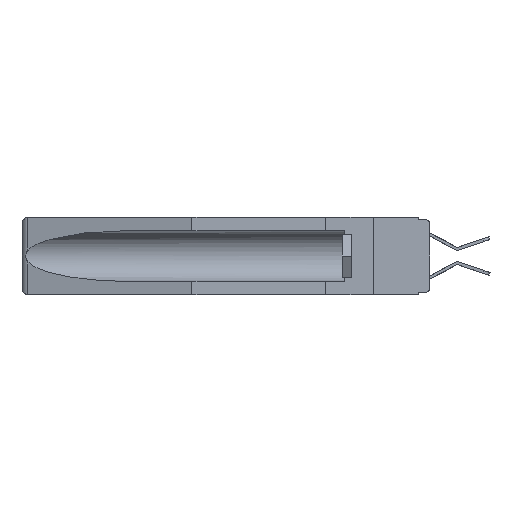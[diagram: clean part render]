
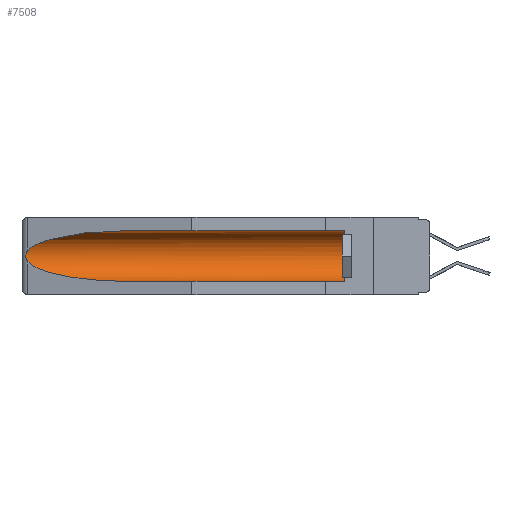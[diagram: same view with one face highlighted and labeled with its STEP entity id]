
A CAD part, left-side view. The second image highlights one B-rep face of the part: STEP entity #7508.
In plain terms, the highlighted cylindrical face has radius 2.857 mm (diameter 5.715 mm), a partial arc.
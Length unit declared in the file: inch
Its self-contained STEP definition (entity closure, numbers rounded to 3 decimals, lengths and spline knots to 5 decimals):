
#489 = CARTESIAN_POINT ( 'NONE',  ( 0.26655, 1.53094, -0.18657 ) ) ;
#800 = VERTEX_POINT ( 'NONE', #11729 ) ;
#881 = CARTESIAN_POINT ( 'NONE',  ( 0.26537, 1.52718, -0.14972 ) ) ;
#1043 = ORIENTED_EDGE ( 'NONE', *, *, #3522, .T. ) ;
#1989 = DIRECTION ( 'NONE',  ( 0., -1., 0. ) ) ;
#3190 = LINE ( 'NONE', #11113, #18363 ) ;
#3226 = CARTESIAN_POINT ( 'NONE',  ( 0.21114, 1.30732, -0.059 ) ) ;
#3404 = CARTESIAN_POINT ( 'NONE',  ( 0.155, 1.07973, -0.284 ) ) ;
#3522 = EDGE_CURVE ( 'NONE', #16618, #800, #25748, .T. ) ;
#3600 = CARTESIAN_POINT ( 'NONE',  ( 0.155, -0.30754, -0.1715 ) ) ;
#3727 = DIRECTION ( 'NONE',  ( 0., 0., 1. ) ) ;
#4139 = CARTESIAN_POINT ( 'NONE',  ( 0.155, 0.126, -0.284 ) ) ;
#4803 = EDGE_CURVE ( 'NONE', #12986, #12432, #3190, .T. ) ;
#4884 = CARTESIAN_POINT ( 'NONE',  ( 0.25451, 1.48313, -0.24835 ) ) ;
#6074 = AXIS2_PLACEMENT_3D ( 'NONE', #23642, #1989, #25483 ) ;
#6491 = CARTESIAN_POINT ( 'NONE',  ( 0.26654, 1.53092, -0.15636 ) ) ;
#6821 = EDGE_LOOP ( 'NONE', ( #10138, #25064, #18909, #18892, #12459, #1043 ) ) ;
#7356 = CARTESIAN_POINT ( 'NONE',  ( 0.155, -0.30754, -0.059 ) ) ;
#7508 = ADVANCED_FACE ( 'NONE', ( #21339 ), #17936, .F. ) ;
#8576 = CARTESIAN_POINT ( 'NONE',  ( 0.26597, 1.5296, -0.19026 ) ) ;
#9327 = CARTESIAN_POINT ( 'NONE',  ( 0.155, 1.07973, -0.059 ) ) ;
#10138 = ORIENTED_EDGE ( 'NONE', *, *, #19722, .T. ) ;
#10212 = CARTESIAN_POINT ( 'NONE',  ( 0.26537, 1.52718, -0.19328 ) ) ;
#11113 = CARTESIAN_POINT ( 'NONE',  ( 0.155, -0.30754, -0.284 ) ) ;
#11729 = CARTESIAN_POINT ( 'NONE',  ( 0.155, 1.07973, -0.059 ) ) ;
#12090 = VECTOR ( 'NONE', #21546, 39.37008 ) ;
#12373 = EDGE_CURVE ( 'NONE', #23852, #12432, #17902, .T. ) ;
#12432 = VERTEX_POINT ( 'NONE', #3404 ) ;
#12459 = ORIENTED_EDGE ( 'NONE', *, *, #13884, .T. ) ;
#12473 = CARTESIAN_POINT ( 'NONE',  ( 0.2675, 1.53308, -0.17534 ) ) ;
#12733 = CARTESIAN_POINT ( 'NONE',  ( 0.2673, 1.5327, -0.16383 ) ) ;
#12986 = VERTEX_POINT ( 'NONE', #4139 ) ;
#13369 = CARTESIAN_POINT ( 'NONE',  ( 0.26537, 1.52718, -0.14972 ) ) ;
#13410 =( BOUNDED_CURVE ( )  B_SPLINE_CURVE ( 3, ( #9327, #3226, #23426, #13369 ),
 .UNSPECIFIED., .F., .F. ) 
 B_SPLINE_CURVE_WITH_KNOTS ( ( 4, 4 ),
 ( 4.71239, 6.08839 ),
 .UNSPECIFIED. ) 
 CURVE ( )  GEOMETRIC_REPRESENTATION_ITEM ( )  RATIONAL_B_SPLINE_CURVE ( ( 1., 0.848, 0.848, 1. ) ) 
 REPRESENTATION_ITEM ( '' )  );
#13884 = EDGE_CURVE ( 'NONE', #12986, #16618, #17296, .T. ) ;
#15513 = AXIS2_PLACEMENT_3D ( 'NONE', #3600, #21589, #3727 ) ;
#15522 = VERTEX_POINT ( 'NONE', #24870 ) ;
#16386 = CARTESIAN_POINT ( 'NONE',  ( 0.2673, 1.53269, -0.17917 ) ) ;
#16521 = CARTESIAN_POINT ( 'NONE',  ( 0.26537, 1.52718, -0.19328 ) ) ;
#16618 = VERTEX_POINT ( 'NONE', #18069 ) ;
#17296 = CIRCLE ( 'NONE', #6074, 0.1125 ) ;
#17902 =( BOUNDED_CURVE ( )  B_SPLINE_CURVE ( 3, ( #23478, #4884, #19177, #23355 ),
 .UNSPECIFIED., .F., .F. ) 
 B_SPLINE_CURVE_WITH_KNOTS ( ( 4, 4 ),
 ( 0.1948, 1.5708 ),
 .UNSPECIFIED. ) 
 CURVE ( )  GEOMETRIC_REPRESENTATION_ITEM ( )  RATIONAL_B_SPLINE_CURVE ( ( 1., 0.848, 0.848, 1. ) ) 
 REPRESENTATION_ITEM ( '' )  );
#17936 = CYLINDRICAL_SURFACE ( 'NONE', #15513, 0.1125 ) ;
#18069 = CARTESIAN_POINT ( 'NONE',  ( 0.155, 0.126, -0.059 ) ) ;
#18363 = VECTOR ( 'NONE', #18832, 39.37008 ) ;
#18742 = CARTESIAN_POINT ( 'NONE',  ( 0.26597, 1.52961, -0.15275 ) ) ;
#18832 = DIRECTION ( 'NONE',  ( 0., 1., 0. ) ) ;
#18892 = ORIENTED_EDGE ( 'NONE', *, *, #4803, .F. ) ;
#18909 = ORIENTED_EDGE ( 'NONE', *, *, #12373, .T. ) ;
#19177 = CARTESIAN_POINT ( 'NONE',  ( 0.21114, 1.30732, -0.284 ) ) ;
#19722 = EDGE_CURVE ( 'NONE', #800, #15522, #13410, .T. ) ;
#20564 = CARTESIAN_POINT ( 'NONE',  ( 0.2675, 1.53308, -0.16763 ) ) ;
#20857 = EDGE_CURVE ( 'NONE', #15522, #23852, #24762, .T. ) ;
#21339 = FACE_OUTER_BOUND ( 'NONE', #6821, .T. ) ;
#21546 = DIRECTION ( 'NONE',  ( 0., 1., 0. ) ) ;
#21589 = DIRECTION ( 'NONE',  ( 0., 1., 0. ) ) ;
#23355 = CARTESIAN_POINT ( 'NONE',  ( 0.155, 1.07973, -0.284 ) ) ;
#23426 = CARTESIAN_POINT ( 'NONE',  ( 0.25451, 1.48313, -0.09465 ) ) ;
#23478 = CARTESIAN_POINT ( 'NONE',  ( 0.26537, 1.52718, -0.19328 ) ) ;
#23642 = CARTESIAN_POINT ( 'NONE',  ( 0.155, 0.126, -0.1715 ) ) ;
#23852 = VERTEX_POINT ( 'NONE', #10212 ) ;
#24762 = B_SPLINE_CURVE_WITH_KNOTS ( 'NONE', 3,
 ( #881, #18742, #6491, #12733, #20564, #12473, #16386, #489, #8576, #16521 ),
 .UNSPECIFIED., .F., .F.,
 ( 4, 2, 2, 2, 4 ),
 ( 0., 0.00029, 0.00058, 0.00087, 0.00117 ),
 .UNSPECIFIED. ) ;
#24870 = CARTESIAN_POINT ( 'NONE',  ( 0.26537, 1.52718, -0.14972 ) ) ;
#25064 = ORIENTED_EDGE ( 'NONE', *, *, #20857, .T. ) ;
#25483 = DIRECTION ( 'NONE',  ( 0., 0., 1. ) ) ;
#25748 = LINE ( 'NONE', #7356, #12090 ) ;
